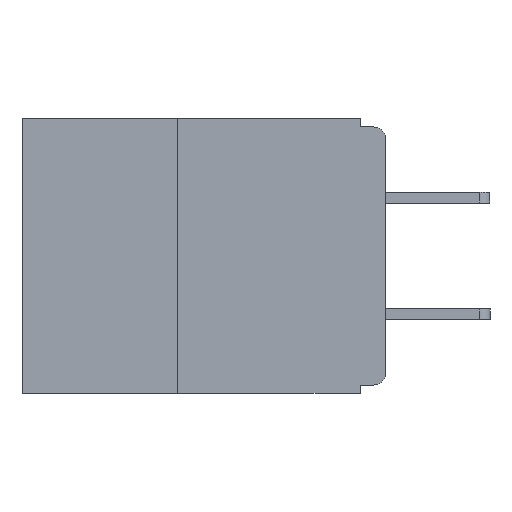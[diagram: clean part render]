
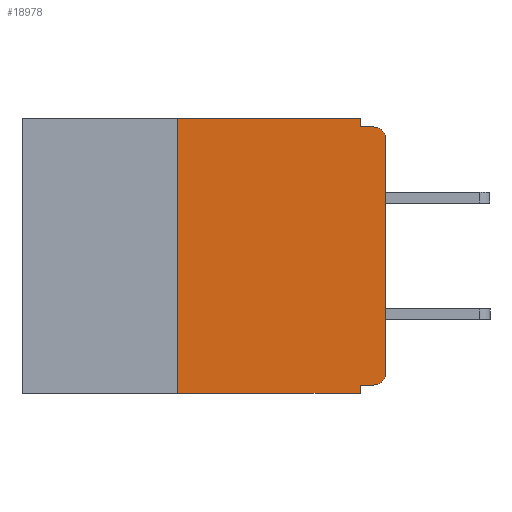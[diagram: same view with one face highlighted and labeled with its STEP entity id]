
A CAD part, left-side view. The second image highlights one B-rep face of the part: STEP entity #18978.
In plain terms, the highlighted planar face has unit normal (-1, 0, 0).
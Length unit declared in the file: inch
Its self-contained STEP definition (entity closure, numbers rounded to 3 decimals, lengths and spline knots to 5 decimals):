
#113 = VERTEX_POINT ( 'NONE', #5334 ) ;
#301 = VERTEX_POINT ( 'NONE', #6340 ) ;
#433 = CARTESIAN_POINT ( 'NONE',  ( 0., 0.031, 0. ) ) ;
#478 = PLANE ( 'NONE',  #20315 ) ;
#588 = VERTEX_POINT ( 'NONE', #18293 ) ;
#1597 = EDGE_CURVE ( 'NONE', #21872, #113, #2942, .T. ) ;
#1694 = CARTESIAN_POINT ( 'NONE',  ( 0., 0.437, -0.33 ) ) ;
#1773 = EDGE_CURVE ( 'NONE', #113, #5250, #13709, .T. ) ;
#2347 = AXIS2_PLACEMENT_3D ( 'NONE', #6515, #18811, #8296 ) ;
#2451 = CARTESIAN_POINT ( 'NONE',  ( 0., 0.031, -0.33 ) ) ;
#2626 = CARTESIAN_POINT ( 'NONE',  ( 0., 0.031, 0. ) ) ;
#2942 = LINE ( 'NONE', #21594, #16472 ) ;
#3017 = CARTESIAN_POINT ( 'NONE',  ( 0., 0., -0.01 ) ) ;
#3749 = CARTESIAN_POINT ( 'NONE',  ( 0., 0.25, -0.33 ) ) ;
#3790 = DIRECTION ( 'NONE',  ( -1., 0., 0. ) ) ;
#3837 = CARTESIAN_POINT ( 'NONE',  ( 0., 0.015, -0.32 ) ) ;
#3944 = DIRECTION ( 'NONE',  ( 0., 1., 0. ) ) ;
#4828 = DIRECTION ( 'NONE',  ( 0., -1., 0. ) ) ;
#4953 = LINE ( 'NONE', #3749, #18461 ) ;
#5163 = DIRECTION ( 'NONE',  ( 0., -1., 0. ) ) ;
#5215 = CARTESIAN_POINT ( 'NONE',  ( 0., 0.015, -0.01 ) ) ;
#5250 = VERTEX_POINT ( 'NONE', #2451 ) ;
#5334 = CARTESIAN_POINT ( 'NONE',  ( 0., 0.031, -0.32 ) ) ;
#5576 = DIRECTION ( 'NONE',  ( 0., 0., 1. ) ) ;
#5626 = ORIENTED_EDGE ( 'NONE', *, *, #19302, .F. ) ;
#5940 = DIRECTION ( 'NONE',  ( 1., 0., 0. ) ) ;
#6114 = LINE ( 'NONE', #8719, #19597 ) ;
#6340 = CARTESIAN_POINT ( 'NONE',  ( 0., 0.25, -0.33 ) ) ;
#6451 = EDGE_CURVE ( 'NONE', #301, #5250, #17616, .T. ) ;
#6515 = CARTESIAN_POINT ( 'NONE',  ( 0., 0.015, -0.025 ) ) ;
#7100 = EDGE_LOOP ( 'NONE', ( #7849, #7365, #5626, #17968, #15971, #13303, #19430, #8878, #14020, #21058 ) ) ;
#7171 = EDGE_CURVE ( 'NONE', #21872, #8869, #17302, .T. ) ;
#7365 = ORIENTED_EDGE ( 'NONE', *, *, #17286, .T. ) ;
#7492 = LINE ( 'NONE', #19786, #16260 ) ;
#7849 = ORIENTED_EDGE ( 'NONE', *, *, #10381, .T. ) ;
#8265 = VECTOR ( 'NONE', #12347, 39.37008 ) ;
#8277 = VECTOR ( 'NONE', #9782, 39.37008 ) ;
#8296 = DIRECTION ( 'NONE',  ( 0., 0., -1. ) ) ;
#8684 = VECTOR ( 'NONE', #4828, 39.37008 ) ;
#8719 = CARTESIAN_POINT ( 'NONE',  ( 0., 0.437, 0. ) ) ;
#8869 = VERTEX_POINT ( 'NONE', #21099 ) ;
#8878 = ORIENTED_EDGE ( 'NONE', *, *, #1773, .F. ) ;
#9064 = VECTOR ( 'NONE', #15497, 39.37008 ) ;
#9287 = CIRCLE ( 'NONE', #2347, 0.015 ) ;
#9782 = DIRECTION ( 'NONE',  ( 0., 0., -1. ) ) ;
#10204 = EDGE_CURVE ( 'NONE', #21822, #11886, #6114, .T. ) ;
#10381 = EDGE_CURVE ( 'NONE', #8869, #19728, #7492, .T. ) ;
#10818 = VERTEX_POINT ( 'NONE', #5215 ) ;
#11116 = CARTESIAN_POINT ( 'NONE',  ( 0., 0.031, -0.33 ) ) ;
#11846 = EDGE_CURVE ( 'NONE', #11886, #588, #22284, .T. ) ;
#11886 = VERTEX_POINT ( 'NONE', #433 ) ;
#12347 = DIRECTION ( 'NONE',  ( 0., -1., 0. ) ) ;
#12580 = CARTESIAN_POINT ( 'NONE',  ( 0., 0.25, 0. ) ) ;
#13121 = CARTESIAN_POINT ( 'NONE',  ( 0., 0., -0.025 ) ) ;
#13303 = ORIENTED_EDGE ( 'NONE', *, *, #15687, .F. ) ;
#13709 = LINE ( 'NONE', #11116, #9064 ) ;
#14020 = ORIENTED_EDGE ( 'NONE', *, *, #1597, .F. ) ;
#14365 = CARTESIAN_POINT ( 'NONE',  ( 0., 0.015, -0.305 ) ) ;
#15497 = DIRECTION ( 'NONE',  ( 0., 0., -1. ) ) ;
#15687 = EDGE_CURVE ( 'NONE', #301, #21822, #4953, .T. ) ;
#15971 = ORIENTED_EDGE ( 'NONE', *, *, #10204, .F. ) ;
#16144 = DIRECTION ( 'NONE',  ( 0., 0., -1. ) ) ;
#16260 = VECTOR ( 'NONE', #21551, 39.37008 ) ;
#16458 = CARTESIAN_POINT ( 'NONE',  ( 0., 0.437, 0. ) ) ;
#16472 = VECTOR ( 'NONE', #3944, 39.37008 ) ;
#17286 = EDGE_CURVE ( 'NONE', #19728, #10818, #9287, .T. ) ;
#17302 = CIRCLE ( 'NONE', #22563, 0.015 ) ;
#17616 = LINE ( 'NONE', #1694, #8265 ) ;
#17968 = ORIENTED_EDGE ( 'NONE', *, *, #11846, .F. ) ;
#18266 = DIRECTION ( 'NONE',  ( 0., 0., -1. ) ) ;
#18293 = CARTESIAN_POINT ( 'NONE',  ( 0., 0.031, -0.01 ) ) ;
#18461 = VECTOR ( 'NONE', #5576, 39.37008 ) ;
#18811 = DIRECTION ( 'NONE',  ( -1., 0., 0. ) ) ;
#18978 = ADVANCED_FACE ( 'NONE', ( #19435 ), #478, .F. ) ;
#19302 = EDGE_CURVE ( 'NONE', #588, #10818, #22697, .T. ) ;
#19430 = ORIENTED_EDGE ( 'NONE', *, *, #6451, .T. ) ;
#19435 = FACE_OUTER_BOUND ( 'NONE', #7100, .T. ) ;
#19597 = VECTOR ( 'NONE', #5163, 39.37008 ) ;
#19728 = VERTEX_POINT ( 'NONE', #13121 ) ;
#19786 = CARTESIAN_POINT ( 'NONE',  ( 0., 0., 0. ) ) ;
#20315 = AXIS2_PLACEMENT_3D ( 'NONE', #16458, #5940, #18266 ) ;
#21058 = ORIENTED_EDGE ( 'NONE', *, *, #7171, .T. ) ;
#21099 = CARTESIAN_POINT ( 'NONE',  ( 0., 0., -0.305 ) ) ;
#21551 = DIRECTION ( 'NONE',  ( 0., 0., 1. ) ) ;
#21594 = CARTESIAN_POINT ( 'NONE',  ( 0., 0., -0.32 ) ) ;
#21822 = VERTEX_POINT ( 'NONE', #12580 ) ;
#21872 = VERTEX_POINT ( 'NONE', #3837 ) ;
#22284 = LINE ( 'NONE', #2626, #8277 ) ;
#22563 = AXIS2_PLACEMENT_3D ( 'NONE', #14365, #3790, #16144 ) ;
#22697 = LINE ( 'NONE', #3017, #8684 ) ;
